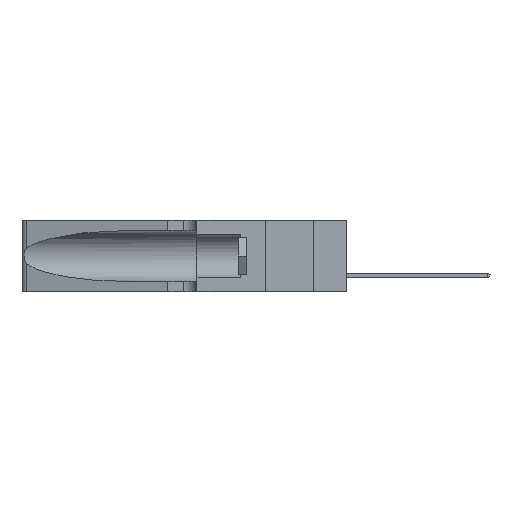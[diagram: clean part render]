
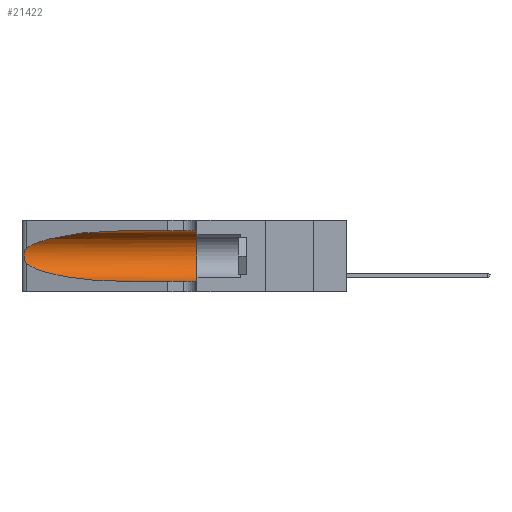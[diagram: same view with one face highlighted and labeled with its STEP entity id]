
A CAD part, left-side view. The second image highlights one B-rep face of the part: STEP entity #21422.
In plain terms, the highlighted cylindrical face has radius 3.308 mm (diameter 6.617 mm), a partial arc.
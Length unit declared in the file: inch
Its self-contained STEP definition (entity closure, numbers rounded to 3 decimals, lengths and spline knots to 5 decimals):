
#547 = EDGE_CURVE ( 'NONE', #7726, #12620, #28950, .T. ) ;
#737 = ORIENTED_EDGE ( 'NONE', *, *, #547, .T. ) ;
#1247 = CARTESIAN_POINT ( 'NONE',  ( 0.25639, 1.23186, 0.15144 ) ) ;
#2358 = CARTESIAN_POINT ( 'NONE',  ( 0.1305, 0.72297, 0.05475 ) ) ;
#2370 = CARTESIAN_POINT ( 'NONE',  ( 0.1305, 1.61858, 0.05475 ) ) ;
#2523 = CARTESIAN_POINT ( 'NONE',  ( 0.18966, 0.96281, 0.05475 ) ) ;
#2936 = CARTESIAN_POINT ( 'NONE',  ( 0.18966, 0.96281, 0.31525 ) ) ;
#3329 = CIRCLE ( 'NONE', #12678, 0.13025 ) ;
#3511 = CARTESIAN_POINT ( 'NONE',  ( 0.25639, 1.23184, 0.21858 ) ) ;
#3627 = CARTESIAN_POINT ( 'NONE',  ( 0.26018, 1.23835, 0.19895 ) ) ;
#3629 = EDGE_CURVE ( 'NONE', #22337, #5179, #3329, .T. ) ;
#5012 = CARTESIAN_POINT ( 'NONE',  ( 0.1305, 0.72297, 0.05475 ) ) ;
#5179 = VERTEX_POINT ( 'NONE', #7107 ) ;
#5308 = ORIENTED_EDGE ( 'NONE', *, *, #14169, .T. ) ;
#5977 = CARTESIAN_POINT ( 'NONE',  ( 0.26075, 1.23896, 0.178 ) ) ;
#7107 = CARTESIAN_POINT ( 'NONE',  ( 0.1305, 0.35, 0.05475 ) ) ;
#7628 = DIRECTION ( 'NONE',  ( 0., -1., 0. ) ) ;
#7726 = VERTEX_POINT ( 'NONE', #30850 ) ;
#8505 = CARTESIAN_POINT ( 'NONE',  ( 0.1305, 0.35, 0.31525 ) ) ;
#9135 = VERTEX_POINT ( 'NONE', #18479 ) ;
#9376 = EDGE_LOOP ( 'NONE', ( #5308, #20170, #737, #12762, #30061, #12386 ) ) ;
#10372 = CARTESIAN_POINT ( 'NONE',  ( 0.25487, 1.22718, 0.22369 ) ) ;
#10943 = CARTESIAN_POINT ( 'NONE',  ( 0.25487, 1.22718, 0.14631 ) ) ;
#11050 = CARTESIAN_POINT ( 'NONE',  ( 0.25555, 1.22993, 0.14849 ) ) ;
#12386 = ORIENTED_EDGE ( 'NONE', *, *, #28966, .F. ) ;
#12620 = VERTEX_POINT ( 'NONE', #2358 ) ;
#12678 = AXIS2_PLACEMENT_3D ( 'NONE', #23593, #18411, #20883 ) ;
#12762 = ORIENTED_EDGE ( 'NONE', *, *, #28216, .T. ) ;
#13300 = CARTESIAN_POINT ( 'NONE',  ( 0.25555, 1.22994, 0.2215 ) ) ;
#13334 = CYLINDRICAL_SURFACE ( 'NONE', #14213, 0.13025 ) ;
#13703 = LINE ( 'NONE', #22020, #24370 ) ;
#14169 = EDGE_CURVE ( 'NONE', #29590, #9135, #17874, .T. ) ;
#14213 = AXIS2_PLACEMENT_3D ( 'NONE', #16182, #31329, #19035 ) ;
#16182 = CARTESIAN_POINT ( 'NONE',  ( 0.1305, 1.61858, 0.185 ) ) ;
#17119 = CARTESIAN_POINT ( 'NONE',  ( 0.25487, 1.22718, 0.14631 ) ) ;
#17406 = CARTESIAN_POINT ( 'NONE',  ( 0.2373, 1.15595, 0.08982 ) ) ;
#17874 =( BOUNDED_CURVE ( )  B_SPLINE_CURVE ( 3, ( #24488, #2936, #25040, #10372 ),
 .UNSPECIFIED., .F., .F. ) 
 B_SPLINE_CURVE_WITH_KNOTS ( ( 4, 4 ),
 ( 1.5708, 2.84003 ),
 .UNSPECIFIED. ) 
 CURVE ( )  GEOMETRIC_REPRESENTATION_ITEM ( )  RATIONAL_B_SPLINE_CURVE ( ( 1., 0.87, 0.87, 1. ) ) 
 REPRESENTATION_ITEM ( '' )  );
#18007 = CARTESIAN_POINT ( 'NONE',  ( 0.1305, 0.72297, 0.31525 ) ) ;
#18411 = DIRECTION ( 'NONE',  ( 0., 1., 0. ) ) ;
#18479 = CARTESIAN_POINT ( 'NONE',  ( 0.25487, 1.22718, 0.22369 ) ) ;
#19035 = DIRECTION ( 'NONE',  ( 0., 0., -1. ) ) ;
#20170 = ORIENTED_EDGE ( 'NONE', *, *, #24094, .T. ) ;
#20646 = CARTESIAN_POINT ( 'NONE',  ( 0.25787, 1.23484, 0.2124 ) ) ;
#20869 = CARTESIAN_POINT ( 'NONE',  ( 0.26075, 1.23896, 0.19203 ) ) ;
#20883 = DIRECTION ( 'NONE',  ( 0., 0., 1. ) ) ;
#21422 = ADVANCED_FACE ( 'NONE', ( #29823 ), #13334, .F. ) ;
#22020 = CARTESIAN_POINT ( 'NONE',  ( 0.1305, 1.61858, 0.31525 ) ) ;
#22337 = VERTEX_POINT ( 'NONE', #8505 ) ;
#22933 = VECTOR ( 'NONE', #7628, 39.37008 ) ;
#23145 = CARTESIAN_POINT ( 'NONE',  ( 0.25789, 1.23486, 0.15765 ) ) ;
#23593 = CARTESIAN_POINT ( 'NONE',  ( 0.1305, 0.35, 0.185 ) ) ;
#23721 = LINE ( 'NONE', #2370, #22933 ) ;
#24094 = EDGE_CURVE ( 'NONE', #9135, #7726, #26565, .T. ) ;
#24370 = VECTOR ( 'NONE', #24585, 39.37008 ) ;
#24488 = CARTESIAN_POINT ( 'NONE',  ( 0.1305, 0.72297, 0.31525 ) ) ;
#24585 = DIRECTION ( 'NONE',  ( 0., -1., 0. ) ) ;
#25040 = CARTESIAN_POINT ( 'NONE',  ( 0.2373, 1.15595, 0.28018 ) ) ;
#25602 = CARTESIAN_POINT ( 'NONE',  ( 0.26017, 1.23833, 0.17102 ) ) ;
#25936 = CARTESIAN_POINT ( 'NONE',  ( 0.25487, 1.22718, 0.22369 ) ) ;
#26565 = B_SPLINE_CURVE_WITH_KNOTS ( 'NONE', 3,
 ( #25936, #13300, #3511, #20646, #30905, #3627, #20869, #5977, #25602, #28424, #23145, #1247, #11050, #10943 ),
 .UNSPECIFIED., .F., .F.,
 ( 4, 2, 2, 2, 2, 2, 4 ),
 ( 0., 0.00027, 0.00053, 0.00107, 0.0016, 0.00187, 0.00214 ),
 .UNSPECIFIED. ) ;
#28216 = EDGE_CURVE ( 'NONE', #12620, #5179, #23721, .T. ) ;
#28424 = CARTESIAN_POINT ( 'NONE',  ( 0.25856, 1.23593, 0.16098 ) ) ;
#28950 =( BOUNDED_CURVE ( )  B_SPLINE_CURVE ( 3, ( #17119, #17406, #2523, #5012 ),
 .UNSPECIFIED., .F., .T. ) 
 B_SPLINE_CURVE_WITH_KNOTS ( ( 4, 4 ),
 ( 3.44316, 4.71239 ),
 .UNSPECIFIED. ) 
 CURVE ( )  GEOMETRIC_REPRESENTATION_ITEM ( )  RATIONAL_B_SPLINE_CURVE ( ( 1., 0.87, 0.87, 1. ) ) 
 REPRESENTATION_ITEM ( '' )  );
#28966 = EDGE_CURVE ( 'NONE', #29590, #22337, #13703, .T. ) ;
#29590 = VERTEX_POINT ( 'NONE', #18007 ) ;
#29823 = FACE_OUTER_BOUND ( 'NONE', #9376, .T. ) ;
#30061 = ORIENTED_EDGE ( 'NONE', *, *, #3629, .F. ) ;
#30850 = CARTESIAN_POINT ( 'NONE',  ( 0.25487, 1.22718, 0.14631 ) ) ;
#30905 = CARTESIAN_POINT ( 'NONE',  ( 0.25854, 1.2359, 0.20912 ) ) ;
#31329 = DIRECTION ( 'NONE',  ( 0., -1., 0. ) ) ;
